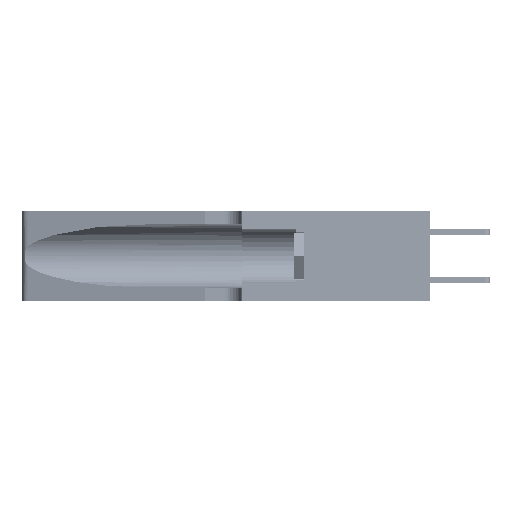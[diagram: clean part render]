
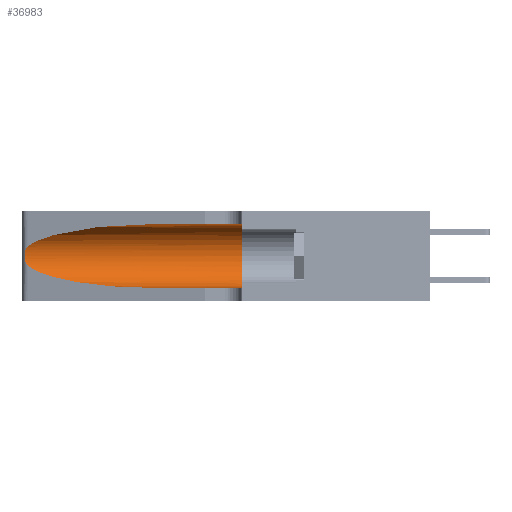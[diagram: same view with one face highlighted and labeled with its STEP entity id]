
A CAD part, left-side view. The second image highlights one B-rep face of the part: STEP entity #36983.
In plain terms, the highlighted cylindrical face has radius 3.308 mm (diameter 6.617 mm), a partial arc.
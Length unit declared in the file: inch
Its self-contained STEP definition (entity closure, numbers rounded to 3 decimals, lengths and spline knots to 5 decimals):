
#29 = CARTESIAN_POINT ( 'NONE',  ( 0.25856, 1.23593, 0.16098 ) ) ;
#182 = VERTEX_POINT ( 'NONE', #14722 ) ;
#2929 = CARTESIAN_POINT ( 'NONE',  ( 0.25555, 1.22994, 0.2215 ) ) ;
#3152 = EDGE_CURVE ( 'NONE', #5407, #27020, #13614, .T. ) ;
#3387 = CARTESIAN_POINT ( 'NONE',  ( 0.1305, 0.35, 0.31525 ) ) ;
#4273 = ORIENTED_EDGE ( 'NONE', *, *, #35668, .T. ) ;
#4302 = CIRCLE ( 'NONE', #42405, 0.13025 ) ;
#4912 = VECTOR ( 'NONE', #34389, 39.37008 ) ;
#5060 = VERTEX_POINT ( 'NONE', #29999 ) ;
#5407 = VERTEX_POINT ( 'NONE', #36085 ) ;
#6274 = CARTESIAN_POINT ( 'NONE',  ( 0.25639, 1.23184, 0.21858 ) ) ;
#9300 = VERTEX_POINT ( 'NONE', #3387 ) ;
#10215 = CARTESIAN_POINT ( 'NONE',  ( 0.25787, 1.23484, 0.2124 ) ) ;
#11263 = DIRECTION ( 'NONE',  ( 0., -1., 0. ) ) ;
#13614 = LINE ( 'NONE', #37406, #4912 ) ;
#14722 = CARTESIAN_POINT ( 'NONE',  ( 0.1305, 0.72297, 0.31525 ) ) ;
#15046 = DIRECTION ( 'NONE',  ( 0., 0., -1. ) ) ;
#15563 = CARTESIAN_POINT ( 'NONE',  ( 0.25487, 1.22718, 0.14631 ) ) ;
#17509 = EDGE_LOOP ( 'NONE', ( #4273, #34620, #26108, #23243, #19925, #39509 ) ) ;
#18705 = CARTESIAN_POINT ( 'NONE',  ( 0.18966, 0.96281, 0.31525 ) ) ;
#19497 = CARTESIAN_POINT ( 'NONE',  ( 0.1305, 0.35, 0.185 ) ) ;
#19925 = ORIENTED_EDGE ( 'NONE', *, *, #44167, .F. ) ;
#20535 = CARTESIAN_POINT ( 'NONE',  ( 0.26075, 1.23896, 0.178 ) ) ;
#21697 = CARTESIAN_POINT ( 'NONE',  ( 0.1305, 1.61858, 0.31525 ) ) ;
#23243 = ORIENTED_EDGE ( 'NONE', *, *, #3152, .T. ) ;
#26108 = ORIENTED_EDGE ( 'NONE', *, *, #41889, .T. ) ;
#26632 = CARTESIAN_POINT ( 'NONE',  ( 0.1305, 0.72297, 0.05475 ) ) ;
#26924 = LINE ( 'NONE', #21697, #31752 ) ;
#27020 = VERTEX_POINT ( 'NONE', #34924 ) ;
#27205 = CARTESIAN_POINT ( 'NONE',  ( 0.25487, 1.22718, 0.14631 ) ) ;
#27353 = CARTESIAN_POINT ( 'NONE',  ( 0.25854, 1.2359, 0.20912 ) ) ;
#27649 = CARTESIAN_POINT ( 'NONE',  ( 0.25555, 1.22993, 0.14849 ) ) ;
#28842 = AXIS2_PLACEMENT_3D ( 'NONE', #32018, #11263, #15046 ) ;
#29707 = B_SPLINE_CURVE_WITH_KNOTS ( 'NONE', 3,
 ( #44512, #2929, #6274, #10215, #27353, #41446, #34175, #20535, #44660, #29, #30532, #44811, #27649, #27205 ),
 .UNSPECIFIED., .F., .F.,
 ( 4, 2, 2, 2, 2, 2, 4 ),
 ( 0., 0.00027, 0.00053, 0.00107, 0.0016, 0.00187, 0.00214 ),
 .UNSPECIFIED. ) ;
#29999 = CARTESIAN_POINT ( 'NONE',  ( 0.25487, 1.22718, 0.22369 ) ) ;
#30532 = CARTESIAN_POINT ( 'NONE',  ( 0.25789, 1.23486, 0.15765 ) ) ;
#31752 = VECTOR ( 'NONE', #35782, 39.37008 ) ;
#32018 = CARTESIAN_POINT ( 'NONE',  ( 0.1305, 1.61858, 0.185 ) ) ;
#32997 = CARTESIAN_POINT ( 'NONE',  ( 0.2373, 1.15595, 0.28018 ) ) ;
#33290 = DIRECTION ( 'NONE',  ( 0., 1., 0. ) ) ;
#33388 = EDGE_CURVE ( 'NONE', #182, #9300, #26924, .T. ) ;
#33844 =( BOUNDED_CURVE ( )  B_SPLINE_CURVE ( 3, ( #15563, #39784, #39954, #26632 ),
 .UNSPECIFIED., .F., .F. ) 
 B_SPLINE_CURVE_WITH_KNOTS ( ( 4, 4 ),
 ( 3.44316, 4.71239 ),
 .UNSPECIFIED. ) 
 CURVE ( )  GEOMETRIC_REPRESENTATION_ITEM ( )  RATIONAL_B_SPLINE_CURVE ( ( 1., 0.87, 0.87, 1. ) ) 
 REPRESENTATION_ITEM ( '' )  );
#34175 = CARTESIAN_POINT ( 'NONE',  ( 0.26075, 1.23896, 0.19203 ) ) ;
#34389 = DIRECTION ( 'NONE',  ( 0., -1., 0. ) ) ;
#34620 = ORIENTED_EDGE ( 'NONE', *, *, #44341, .T. ) ;
#34924 = CARTESIAN_POINT ( 'NONE',  ( 0.1305, 0.35, 0.05475 ) ) ;
#35668 = EDGE_CURVE ( 'NONE', #182, #5060, #35773, .T. ) ;
#35773 =( BOUNDED_CURVE ( )  B_SPLINE_CURVE ( 3, ( #43322, #18705, #32997, #43480 ),
 .UNSPECIFIED., .F., .T. ) 
 B_SPLINE_CURVE_WITH_KNOTS ( ( 4, 4 ),
 ( 1.5708, 2.84003 ),
 .UNSPECIFIED. ) 
 CURVE ( )  GEOMETRIC_REPRESENTATION_ITEM ( )  RATIONAL_B_SPLINE_CURVE ( ( 1., 0.87, 0.87, 1. ) ) 
 REPRESENTATION_ITEM ( '' )  );
#35782 = DIRECTION ( 'NONE',  ( 0., -1., 0. ) ) ;
#36085 = CARTESIAN_POINT ( 'NONE',  ( 0.1305, 0.72297, 0.05475 ) ) ;
#36983 = ADVANCED_FACE ( 'NONE', ( #42349 ), #37992, .F. ) ;
#37045 = DIRECTION ( 'NONE',  ( 0., 0., 1. ) ) ;
#37406 = CARTESIAN_POINT ( 'NONE',  ( 0.1305, 1.61858, 0.05475 ) ) ;
#37992 = CYLINDRICAL_SURFACE ( 'NONE', #28842, 0.13025 ) ;
#39509 = ORIENTED_EDGE ( 'NONE', *, *, #33388, .F. ) ;
#39784 = CARTESIAN_POINT ( 'NONE',  ( 0.2373, 1.15595, 0.08982 ) ) ;
#39954 = CARTESIAN_POINT ( 'NONE',  ( 0.18966, 0.96281, 0.05475 ) ) ;
#40084 = VERTEX_POINT ( 'NONE', #44375 ) ;
#41446 = CARTESIAN_POINT ( 'NONE',  ( 0.26018, 1.23835, 0.19895 ) ) ;
#41889 = EDGE_CURVE ( 'NONE', #40084, #5407, #33844, .T. ) ;
#42349 = FACE_OUTER_BOUND ( 'NONE', #17509, .T. ) ;
#42405 = AXIS2_PLACEMENT_3D ( 'NONE', #19497, #33290, #37045 ) ;
#43322 = CARTESIAN_POINT ( 'NONE',  ( 0.1305, 0.72297, 0.31525 ) ) ;
#43480 = CARTESIAN_POINT ( 'NONE',  ( 0.25487, 1.22718, 0.22369 ) ) ;
#44167 = EDGE_CURVE ( 'NONE', #9300, #27020, #4302, .T. ) ;
#44341 = EDGE_CURVE ( 'NONE', #5060, #40084, #29707, .T. ) ;
#44375 = CARTESIAN_POINT ( 'NONE',  ( 0.25487, 1.22718, 0.14631 ) ) ;
#44512 = CARTESIAN_POINT ( 'NONE',  ( 0.25487, 1.22718, 0.22369 ) ) ;
#44660 = CARTESIAN_POINT ( 'NONE',  ( 0.26017, 1.23833, 0.17102 ) ) ;
#44811 = CARTESIAN_POINT ( 'NONE',  ( 0.25639, 1.23186, 0.15144 ) ) ;
